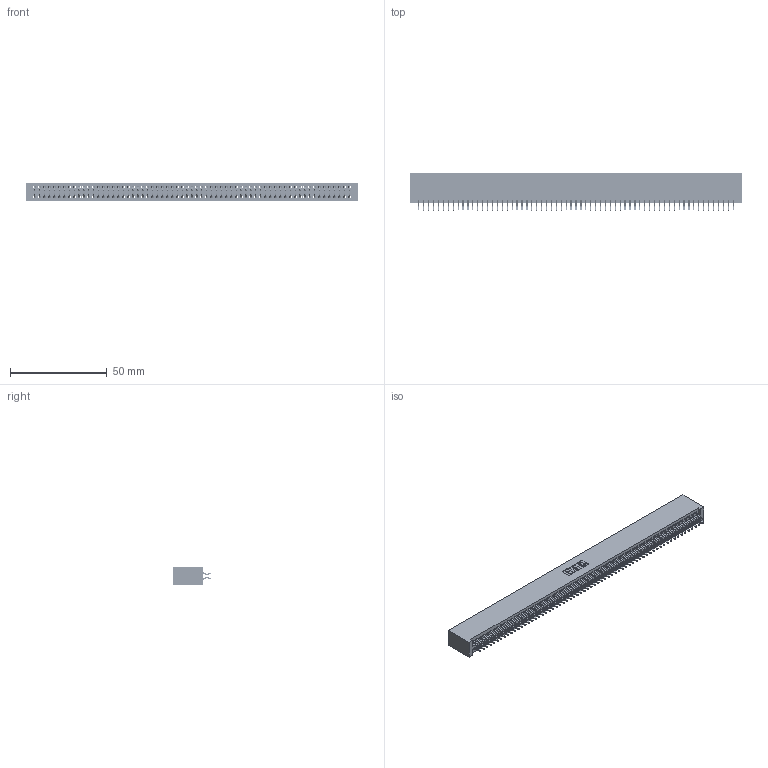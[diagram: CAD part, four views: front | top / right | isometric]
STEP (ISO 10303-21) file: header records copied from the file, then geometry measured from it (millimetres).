
FILE_DESCRIPTION (( 'STEP AP203' ), '1' );
FILE_NAME ('395-130-556-201.STEP', '2018-12-04T19:04:54', ( '' ), ( '' ), 'SwSTEP 2.0', 'SolidWorks 2016', '' );
FILE_SCHEMA (( 'CONFIG_CONTROL_DESIGN' ));
Length unit declared in the file: inch
Products named in the file (3): 395-130-556-201; 345 Part_No Mounting Lugs; 345-292-001_556 Tail
Assembly tree (131 placements, depth 2):
  395-130-556-201
    345 Part_No Mounting Lugs
    345-292-001_556 Tail  x130
Bounding box: 171.7 x 19.24 x 9.4 mm (x, y, z)
Volume: 17503.8 mm3; surface area: 26508.4 mm2
Topology: 131 solids, 131 shells, 7398 faces, 22027 edges, 14510 vertices
Faces by surface type: plane 4886, cylinder 2512
Entity records: 47847 total; most frequent: CARTESIAN_POINT 8012, ORIENTED_EDGE 7934, DIRECTION 7019, EDGE_CURVE 3967, VECTOR 3575, LINE 3575, VERTEX_POINT 2642, AXIS2_PLACEMENT_3D 1722
